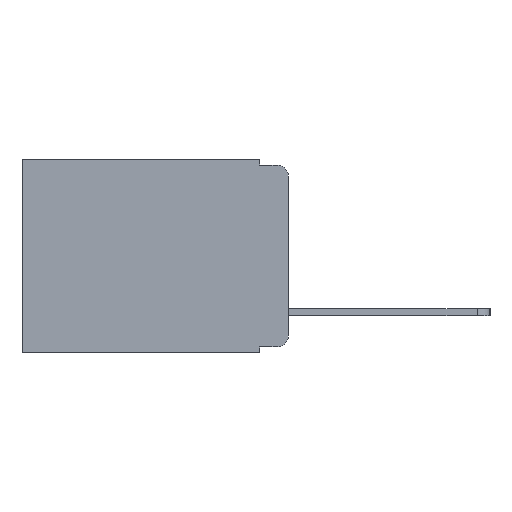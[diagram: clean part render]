
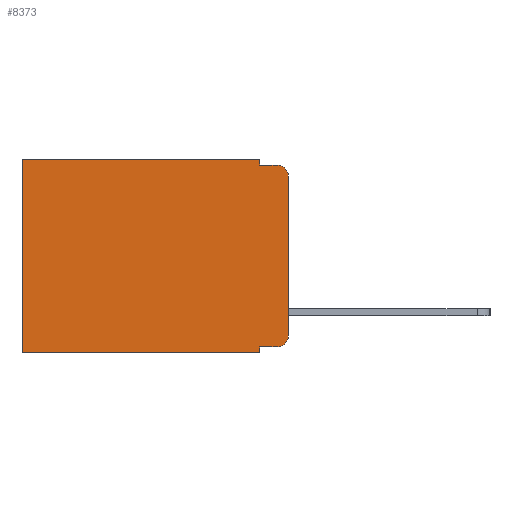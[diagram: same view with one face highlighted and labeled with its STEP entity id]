
A CAD part, left-side view. The second image highlights one B-rep face of the part: STEP entity #8373.
In plain terms, the highlighted planar face has unit normal (-1, 0, 0).
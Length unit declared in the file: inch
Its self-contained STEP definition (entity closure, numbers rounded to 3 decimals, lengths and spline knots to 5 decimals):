
#6 = VECTOR ( 'NONE', #7324, 39.37008 ) ;
#7 = DIRECTION ( 'NONE',  ( 0., 0., -1. ) ) ;
#528 = ORIENTED_EDGE ( 'NONE', *, *, #13779, .T. ) ;
#716 = VECTOR ( 'NONE', #7, 39.37008 ) ;
#1295 = CARTESIAN_POINT ( 'NONE',  ( 0.298, 0.051, 0. ) ) ;
#1701 = CARTESIAN_POINT ( 'NONE',  ( 0.298, 0.051, -0.343 ) ) ;
#1943 = CARTESIAN_POINT ( 'NONE',  ( 0.298, 0.02, -0.01 ) ) ;
#2585 = DIRECTION ( 'NONE',  ( 0., 0., -1. ) ) ;
#2671 = EDGE_CURVE ( 'NONE', #5695, #9263, #6687, .T. ) ;
#3176 = ORIENTED_EDGE ( 'NONE', *, *, #11147, .T. ) ;
#3242 = VERTEX_POINT ( 'NONE', #15734 ) ;
#3658 = EDGE_CURVE ( 'NONE', #9263, #3968, #15766, .T. ) ;
#3815 = CARTESIAN_POINT ( 'NONE',  ( 0.298, 0.02, -0.03 ) ) ;
#3968 = VERTEX_POINT ( 'NONE', #1943 ) ;
#4265 = CARTESIAN_POINT ( 'NONE',  ( 0.298, 0.051, -0.01 ) ) ;
#4358 = EDGE_CURVE ( 'NONE', #5268, #13484, #11148, .T. ) ;
#5226 = DIRECTION ( 'NONE',  ( 0., 0., -1. ) ) ;
#5268 = VERTEX_POINT ( 'NONE', #7126 ) ;
#5523 = VECTOR ( 'NONE', #12051, 39.37008 ) ;
#5695 = VERTEX_POINT ( 'NONE', #7977 ) ;
#5746 = PLANE ( 'NONE',  #11713 ) ;
#5896 = CARTESIAN_POINT ( 'NONE',  ( 0.298, 0., 0. ) ) ;
#6016 = ORIENTED_EDGE ( 'NONE', *, *, #15380, .F. ) ;
#6091 = AXIS2_PLACEMENT_3D ( 'NONE', #16519, #8489, #17772 ) ;
#6129 = CARTESIAN_POINT ( 'NONE',  ( 0.298, 0., 0. ) ) ;
#6241 = CARTESIAN_POINT ( 'NONE',  ( 0.298, 0., -0.03 ) ) ;
#6687 = LINE ( 'NONE', #1295, #17061 ) ;
#7126 = CARTESIAN_POINT ( 'NONE',  ( 0.298, 0.051, -0.333 ) ) ;
#7174 = CARTESIAN_POINT ( 'NONE',  ( 0.298, 0., 0. ) ) ;
#7214 = VERTEX_POINT ( 'NONE', #17066 ) ;
#7324 = DIRECTION ( 'NONE',  ( 0., 1., 0. ) ) ;
#7352 = DIRECTION ( 'NONE',  ( 0., 1., 0. ) ) ;
#7358 = ORIENTED_EDGE ( 'NONE', *, *, #11261, .T. ) ;
#7977 = CARTESIAN_POINT ( 'NONE',  ( 0.298, 0.051, 0. ) ) ;
#8269 = VECTOR ( 'NONE', #10361, 39.37008 ) ;
#8271 = AXIS2_PLACEMENT_3D ( 'NONE', #3815, #13420, #5226 ) ;
#8302 = LINE ( 'NONE', #14083, #14998 ) ;
#8373 = ADVANCED_FACE ( 'NONE', ( #17131 ), #5746, .F. ) ;
#8489 = DIRECTION ( 'NONE',  ( -1., 0., 0. ) ) ;
#8603 = DIRECTION ( 'NONE',  ( 0., 0., -1. ) ) ;
#8666 = VECTOR ( 'NONE', #14056, 39.37008 ) ;
#8784 = EDGE_CURVE ( 'NONE', #17813, #3242, #14396, .T. ) ;
#9263 = VERTEX_POINT ( 'NONE', #4265 ) ;
#9362 = EDGE_CURVE ( 'NONE', #13484, #7214, #8302, .T. ) ;
#9370 = CARTESIAN_POINT ( 'NONE',  ( 0.298, 0.051, -0.333 ) ) ;
#9743 = ORIENTED_EDGE ( 'NONE', *, *, #11935, .T. ) ;
#10361 = DIRECTION ( 'NONE',  ( 0., 0., -1. ) ) ;
#10761 = CARTESIAN_POINT ( 'NONE',  ( 0.298, 0.473, 0. ) ) ;
#11116 = CIRCLE ( 'NONE', #8271, 0.02 ) ;
#11147 = EDGE_CURVE ( 'NONE', #5695, #17241, #15741, .T. ) ;
#11148 = LINE ( 'NONE', #15354, #716 ) ;
#11181 = CARTESIAN_POINT ( 'NONE',  ( 0.298, 0.473, 0. ) ) ;
#11261 = EDGE_CURVE ( 'NONE', #17241, #7214, #16379, .T. ) ;
#11394 = EDGE_LOOP ( 'NONE', ( #6016, #9743, #16851, #17225, #3176, #7358, #14512, #14938, #528, #15370 ) ) ;
#11713 = AXIS2_PLACEMENT_3D ( 'NONE', #7174, #16638, #8603 ) ;
#11818 = LINE ( 'NONE', #6129, #8269 ) ;
#11867 = VECTOR ( 'NONE', #17323, 39.37008 ) ;
#11935 = EDGE_CURVE ( 'NONE', #12676, #3968, #11116, .T. ) ;
#12051 = DIRECTION ( 'NONE',  ( 0., 0., -1. ) ) ;
#12676 = VERTEX_POINT ( 'NONE', #6241 ) ;
#12794 = CARTESIAN_POINT ( 'NONE',  ( 0.298, 0.02, -0.333 ) ) ;
#13420 = DIRECTION ( 'NONE',  ( -1., 0., 0. ) ) ;
#13484 = VERTEX_POINT ( 'NONE', #1701 ) ;
#13779 = EDGE_CURVE ( 'NONE', #5268, #17813, #16301, .T. ) ;
#14056 = DIRECTION ( 'NONE',  ( 0., -1., 0. ) ) ;
#14083 = CARTESIAN_POINT ( 'NONE',  ( 0.298, 0., -0.343 ) ) ;
#14396 = CIRCLE ( 'NONE', #6091, 0.02 ) ;
#14512 = ORIENTED_EDGE ( 'NONE', *, *, #9362, .F. ) ;
#14938 = ORIENTED_EDGE ( 'NONE', *, *, #4358, .F. ) ;
#14998 = VECTOR ( 'NONE', #7352, 39.37008 ) ;
#15354 = CARTESIAN_POINT ( 'NONE',  ( 0.298, 0.051, 0. ) ) ;
#15370 = ORIENTED_EDGE ( 'NONE', *, *, #8784, .T. ) ;
#15380 = EDGE_CURVE ( 'NONE', #12676, #3242, #11818, .T. ) ;
#15734 = CARTESIAN_POINT ( 'NONE',  ( 0.298, 0., -0.313 ) ) ;
#15741 = LINE ( 'NONE', #5896, #6 ) ;
#15766 = LINE ( 'NONE', #16496, #8666 ) ;
#16301 = LINE ( 'NONE', #9370, #11867 ) ;
#16379 = LINE ( 'NONE', #10761, #5523 ) ;
#16496 = CARTESIAN_POINT ( 'NONE',  ( 0.298, 0.051, -0.01 ) ) ;
#16519 = CARTESIAN_POINT ( 'NONE',  ( 0.298, 0.02, -0.313 ) ) ;
#16638 = DIRECTION ( 'NONE',  ( 1., 0., 0. ) ) ;
#16851 = ORIENTED_EDGE ( 'NONE', *, *, #3658, .F. ) ;
#17061 = VECTOR ( 'NONE', #2585, 39.37008 ) ;
#17066 = CARTESIAN_POINT ( 'NONE',  ( 0.298, 0.473, -0.343 ) ) ;
#17131 = FACE_OUTER_BOUND ( 'NONE', #11394, .T. ) ;
#17225 = ORIENTED_EDGE ( 'NONE', *, *, #2671, .F. ) ;
#17241 = VERTEX_POINT ( 'NONE', #11181 ) ;
#17323 = DIRECTION ( 'NONE',  ( 0., -1., 0. ) ) ;
#17772 = DIRECTION ( 'NONE',  ( 0., 0., -1. ) ) ;
#17813 = VERTEX_POINT ( 'NONE', #12794 ) ;
